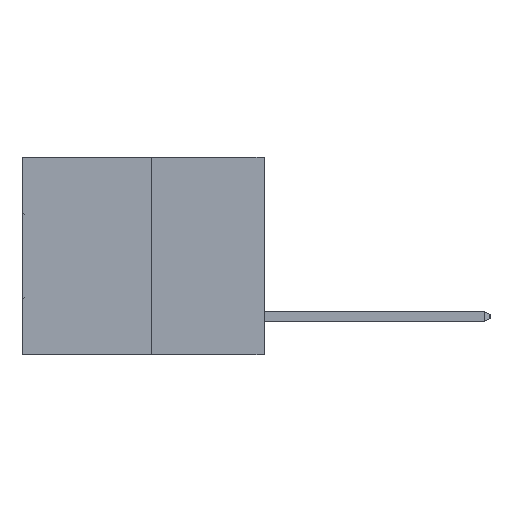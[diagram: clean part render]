
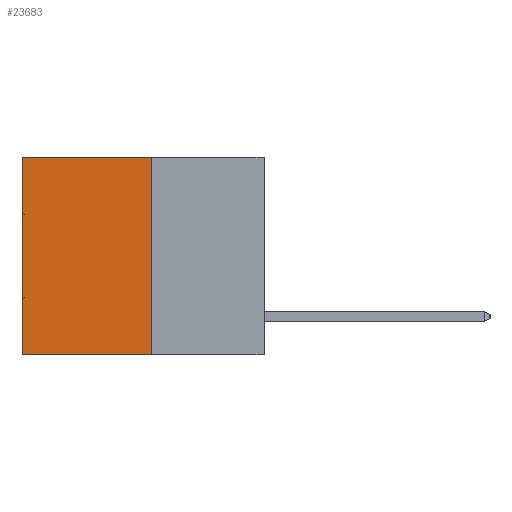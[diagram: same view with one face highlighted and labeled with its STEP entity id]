
A CAD part, left-side view. The second image highlights one B-rep face of the part: STEP entity #23683.
In plain terms, the highlighted planar face has unit normal (-1, 0, 0).
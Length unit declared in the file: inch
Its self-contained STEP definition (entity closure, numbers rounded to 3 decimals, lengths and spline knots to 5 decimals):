
#17 = CARTESIAN_POINT ( 'NONE',  ( 0.3165, 0.6, 0. ) ) ;
#1159 = EDGE_CURVE ( 'NONE', #16668, #17796, #17674, .T. ) ;
#1386 = ORIENTED_EDGE ( 'NONE', *, *, #10343, .T. ) ;
#2013 = VERTEX_POINT ( 'NONE', #17473 ) ;
#2237 = CARTESIAN_POINT ( 'NONE',  ( 0.3165, 0.28, -0.49 ) ) ;
#2294 = FACE_OUTER_BOUND ( 'NONE', #32453, .T. ) ;
#2351 = LINE ( 'NONE', #6291, #3581 ) ;
#2662 = DIRECTION ( 'NONE',  ( 0., 0., -1. ) ) ;
#3581 = VECTOR ( 'NONE', #4351, 39.37008 ) ;
#4351 = DIRECTION ( 'NONE',  ( 0., 1., 0. ) ) ;
#6067 = CARTESIAN_POINT ( 'NONE',  ( 0.3165, 0.28, -0.49 ) ) ;
#6291 = CARTESIAN_POINT ( 'NONE',  ( 0.3165, 0.28, -0.49 ) ) ;
#9192 = EDGE_CURVE ( 'NONE', #11253, #17796, #2351, .T. ) ;
#9906 = CARTESIAN_POINT ( 'NONE',  ( 0.3165, 0.28, 0. ) ) ;
#10343 = EDGE_CURVE ( 'NONE', #2013, #16668, #26418, .T. ) ;
#10606 = ORIENTED_EDGE ( 'NONE', *, *, #1159, .T. ) ;
#10722 = VECTOR ( 'NONE', #2662, 39.37008 ) ;
#11253 = VERTEX_POINT ( 'NONE', #29112 ) ;
#12113 = LINE ( 'NONE', #2237, #32206 ) ;
#12126 = VECTOR ( 'NONE', #20751, 39.37008 ) ;
#15259 = ORIENTED_EDGE ( 'NONE', *, *, #17651, .F. ) ;
#15310 = CARTESIAN_POINT ( 'NONE',  ( 0.3165, 0.6, -0.49 ) ) ;
#16668 = VERTEX_POINT ( 'NONE', #17 ) ;
#17473 = CARTESIAN_POINT ( 'NONE',  ( 0.3165, 0.28, 0. ) ) ;
#17651 = EDGE_CURVE ( 'NONE', #2013, #11253, #12113, .T. ) ;
#17674 = LINE ( 'NONE', #15310, #10722 ) ;
#17796 = VERTEX_POINT ( 'NONE', #19457 ) ;
#19401 = PLANE ( 'NONE',  #20805 ) ;
#19457 = CARTESIAN_POINT ( 'NONE',  ( 0.3165, 0.6, -0.49 ) ) ;
#20751 = DIRECTION ( 'NONE',  ( 0., 1., 0. ) ) ;
#20805 = AXIS2_PLACEMENT_3D ( 'NONE', #6067, #29611, #30050 ) ;
#21528 = ORIENTED_EDGE ( 'NONE', *, *, #9192, .F. ) ;
#23683 = ADVANCED_FACE ( 'NONE', ( #2294 ), #19401, .F. ) ;
#26418 = LINE ( 'NONE', #9906, #12126 ) ;
#29112 = CARTESIAN_POINT ( 'NONE',  ( 0.3165, 0.28, -0.49 ) ) ;
#29611 = DIRECTION ( 'NONE',  ( 1., 0., 0. ) ) ;
#30050 = DIRECTION ( 'NONE',  ( 0., 0., -1. ) ) ;
#32206 = VECTOR ( 'NONE', #33673, 39.37008 ) ;
#32453 = EDGE_LOOP ( 'NONE', ( #10606, #21528, #15259, #1386 ) ) ;
#33673 = DIRECTION ( 'NONE',  ( 0., 0., -1. ) ) ;
